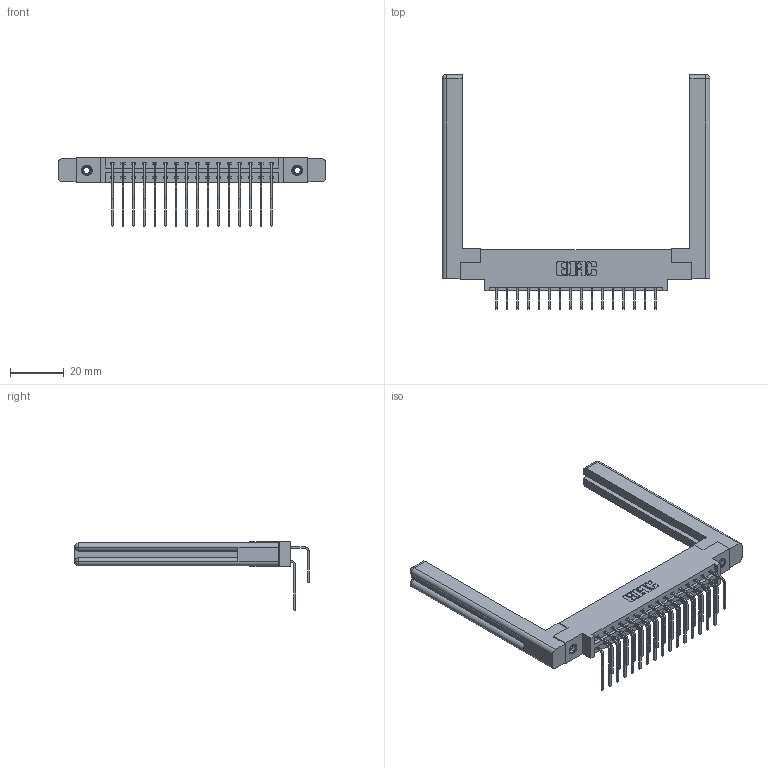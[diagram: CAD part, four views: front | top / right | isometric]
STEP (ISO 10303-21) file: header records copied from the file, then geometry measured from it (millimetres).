
FILE_DESCRIPTION (( 'STEP AP203' ), '1' );
FILE_NAME ('337-032-558-858.STEP', '2019-10-11T01:15:26', ( '' ), ( '' ), 'SwSTEP 2.0', 'SolidWorks 2016', '' );
FILE_SCHEMA (( 'CONFIG_CONTROL_DESIGN' ));
Length unit declared in the file: inch
Products named in the file (6): 345-250-001_345-250-001-102; 307-220-058; 345-292-001_558 559 Tail - 1; 337 Part_0.170 Offset - 0.156 Dia-TI; 337-032-558-858; 345-292-001_558 Tail - 2
Assembly tree (37 placements, depth 2):
  337-032-558-858
    337 Part_0.170 Offset - 0.156 Dia-TI
    345-292-001_558 559 Tail - 1  x16
    345-292-001_558 Tail - 2  x16
    345-250-001_345-250-001-102  x2
    307-220-058  x2
Bounding box: 100.03 x 87.57 x 25.53 mm (x, y, z)
Volume: 17404.8 mm3; surface area: 17430.7 mm2
Topology: 37 solids, 37 shells, 2052 faces, 6021 edges, 3958 vertices
Faces by surface type: plane 1438, cylinder 590, cone 12, torus 12
Entity records: 20318 total; most frequent: CARTESIAN_POINT 3500, ORIENTED_EDGE 3324, DIRECTION 3022, EDGE_CURVE 1662, LINE 1446, VECTOR 1446, VERTEX_POINT 1098, AXIS2_PLACEMENT_3D 788
